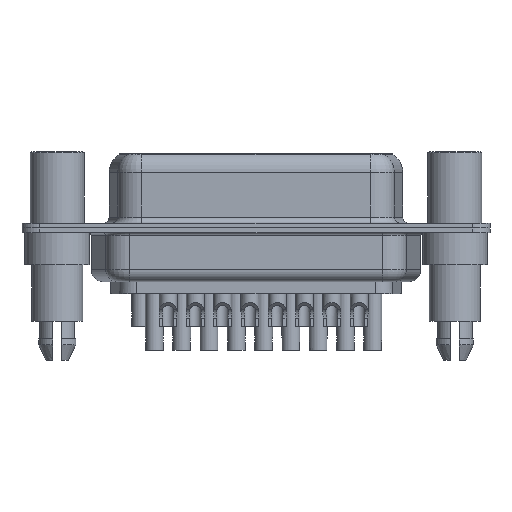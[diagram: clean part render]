
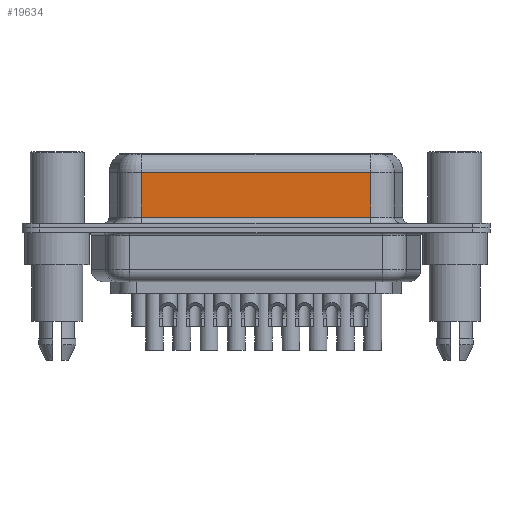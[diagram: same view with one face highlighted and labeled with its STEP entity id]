
A CAD part, front view. The second image highlights one B-rep face of the part: STEP entity #19634.
In plain terms, the highlighted planar face has unit normal (0, -1, 0).
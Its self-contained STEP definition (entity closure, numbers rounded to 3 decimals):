
#2142 = VERTEX_POINT ( 'NONE', #5232 ) ;
#3113 = VECTOR ( 'NONE', #15749, 1000. ) ;
#4042 = CARTESIAN_POINT ( 'NONE',  ( 26.262, -3.95, 4.65 ) ) ;
#4473 = DIRECTION ( 'NONE',  ( 0., 0., -1. ) ) ;
#4709 = AXIS2_PLACEMENT_3D ( 'NONE', #15606, #15855, #21193 ) ;
#5196 = EDGE_CURVE ( 'NONE', #7350, #12186, #23339, .T. ) ;
#5232 = CARTESIAN_POINT ( 'NONE',  ( 26.262, -3.95, 4.65 ) ) ;
#5695 = ORIENTED_EDGE ( 'NONE', *, *, #20279, .F. ) ;
#5998 = VERTEX_POINT ( 'NONE', #13817 ) ;
#6237 = CARTESIAN_POINT ( 'NONE',  ( 26.262, -3.95, 0.9 ) ) ;
#7350 = VERTEX_POINT ( 'NONE', #16279 ) ;
#7462 = ORIENTED_EDGE ( 'NONE', *, *, #5196, .T. ) ;
#9258 = VECTOR ( 'NONE', #12008, 1000. ) ;
#10127 = FACE_OUTER_BOUND ( 'NONE', #16383, .T. ) ;
#10275 = CARTESIAN_POINT ( 'NONE',  ( 26.262, -3.95, 0.9 ) ) ;
#10282 = LINE ( 'NONE', #4042, #3113 ) ;
#12008 = DIRECTION ( 'NONE',  ( 1., 0., 0. ) ) ;
#12186 = VERTEX_POINT ( 'NONE', #6237 ) ;
#12415 = DIRECTION ( 'NONE',  ( 0., 0., -1. ) ) ;
#13461 = VECTOR ( 'NONE', #12415, 1000. ) ;
#13613 = PLANE ( 'NONE',  #4709 ) ;
#13817 = CARTESIAN_POINT ( 'NONE',  ( 7.038, -3.95, 4.65 ) ) ;
#13945 = LINE ( 'NONE', #21518, #18607 ) ;
#15606 = CARTESIAN_POINT ( 'NONE',  ( 26.262, -3.95, 6.4 ) ) ;
#15749 = DIRECTION ( 'NONE',  ( -1., 0., 0. ) ) ;
#15855 = DIRECTION ( 'NONE',  ( 0., 1., 0. ) ) ;
#16231 = EDGE_CURVE ( 'NONE', #5998, #7350, #13945, .T. ) ;
#16279 = CARTESIAN_POINT ( 'NONE',  ( 7.038, -3.95, 0.9 ) ) ;
#16383 = EDGE_LOOP ( 'NONE', ( #5695, #20632, #23751, #7462 ) ) ;
#16390 = LINE ( 'NONE', #18498, #13461 ) ;
#18498 = CARTESIAN_POINT ( 'NONE',  ( 26.262, -3.95, 6.4 ) ) ;
#18607 = VECTOR ( 'NONE', #4473, 1000. ) ;
#19183 = EDGE_CURVE ( 'NONE', #2142, #5998, #10282, .T. ) ;
#19634 = ADVANCED_FACE ( 'NONE', ( #10127 ), #13613, .F. ) ;
#20279 = EDGE_CURVE ( 'NONE', #2142, #12186, #16390, .T. ) ;
#20632 = ORIENTED_EDGE ( 'NONE', *, *, #19183, .T. ) ;
#21193 = DIRECTION ( 'NONE',  ( -1., 0., 0. ) ) ;
#21518 = CARTESIAN_POINT ( 'NONE',  ( 7.038, -3.95, 6.4 ) ) ;
#23339 = LINE ( 'NONE', #10275, #9258 ) ;
#23751 = ORIENTED_EDGE ( 'NONE', *, *, #16231, .T. ) ;
